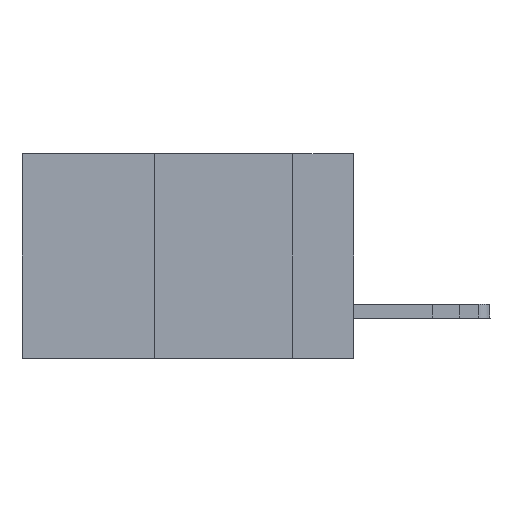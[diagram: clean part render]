
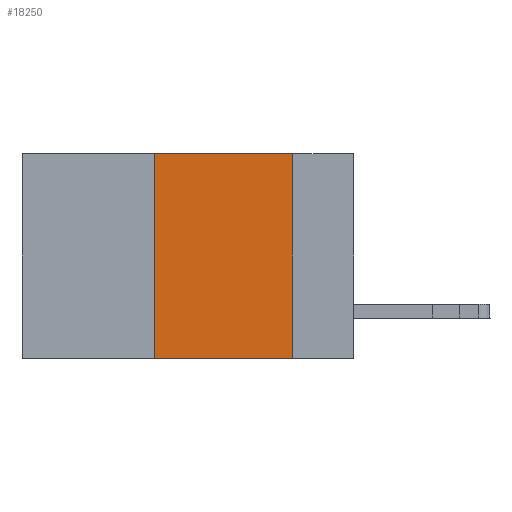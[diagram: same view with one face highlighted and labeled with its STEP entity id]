
A CAD part, left-side view. The second image highlights one B-rep face of the part: STEP entity #18250.
In plain terms, the highlighted planar face has unit normal (-1, 0, 0).
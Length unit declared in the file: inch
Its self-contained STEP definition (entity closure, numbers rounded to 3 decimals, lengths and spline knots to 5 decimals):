
#1842 = AXIS2_PLACEMENT_3D ( 'NONE', #34913, #21122, #20950 ) ;
#3930 = EDGE_CURVE ( 'NONE', #26078, #7096, #12836, .T. ) ;
#4949 = EDGE_CURVE ( 'NONE', #15551, #18416, #33529, .T. ) ;
#5114 = VECTOR ( 'NONE', #28613, 39.37008 ) ;
#7096 = VERTEX_POINT ( 'NONE', #31256 ) ;
#7903 = CARTESIAN_POINT ( 'NONE',  ( 0., 0.11, 0. ) ) ;
#8027 = VECTOR ( 'NONE', #15984, 39.37008 ) ;
#8038 = ORIENTED_EDGE ( 'NONE', *, *, #3930, .T. ) ;
#12127 = CARTESIAN_POINT ( 'NONE',  ( 0., 0.6, -0.37 ) ) ;
#12376 = DIRECTION ( 'NONE',  ( 0., 0., -1. ) ) ;
#12836 = LINE ( 'NONE', #12127, #24693 ) ;
#13246 = EDGE_LOOP ( 'NONE', ( #24107, #16454, #21526, #8038 ) ) ;
#15439 = CARTESIAN_POINT ( 'NONE',  ( 0., 0.11, 0. ) ) ;
#15551 = VERTEX_POINT ( 'NONE', #26642 ) ;
#15674 = PLANE ( 'NONE',  #1842 ) ;
#15984 = DIRECTION ( 'NONE',  ( 0., 0., 1. ) ) ;
#16454 = ORIENTED_EDGE ( 'NONE', *, *, #4949, .F. ) ;
#17394 = EDGE_CURVE ( 'NONE', #18416, #7096, #20714, .T. ) ;
#18250 = ADVANCED_FACE ( 'NONE', ( #31827 ), #15674, .F. ) ;
#18416 = VERTEX_POINT ( 'NONE', #7903 ) ;
#18526 = LINE ( 'NONE', #27226, #8027 ) ;
#20714 = LINE ( 'NONE', #15439, #32490 ) ;
#20950 = DIRECTION ( 'NONE',  ( 0., 0., -1. ) ) ;
#21122 = DIRECTION ( 'NONE',  ( 1., 0., 0. ) ) ;
#21526 = ORIENTED_EDGE ( 'NONE', *, *, #27087, .F. ) ;
#23174 = DIRECTION ( 'NONE',  ( 0., -1., 0. ) ) ;
#24107 = ORIENTED_EDGE ( 'NONE', *, *, #17394, .F. ) ;
#24693 = VECTOR ( 'NONE', #23174, 39.37008 ) ;
#25919 = CARTESIAN_POINT ( 'NONE',  ( 0., 0.36, -0.37 ) ) ;
#26078 = VERTEX_POINT ( 'NONE', #25919 ) ;
#26642 = CARTESIAN_POINT ( 'NONE',  ( 0., 0.36, 0. ) ) ;
#27087 = EDGE_CURVE ( 'NONE', #26078, #15551, #18526, .T. ) ;
#27226 = CARTESIAN_POINT ( 'NONE',  ( 0., 0.36, 0. ) ) ;
#28613 = DIRECTION ( 'NONE',  ( 0., -1., 0. ) ) ;
#30978 = CARTESIAN_POINT ( 'NONE',  ( 0., 0.6, 0. ) ) ;
#31256 = CARTESIAN_POINT ( 'NONE',  ( 0., 0.11, -0.37 ) ) ;
#31827 = FACE_OUTER_BOUND ( 'NONE', #13246, .T. ) ;
#32490 = VECTOR ( 'NONE', #12376, 39.37008 ) ;
#33529 = LINE ( 'NONE', #30978, #5114 ) ;
#34913 = CARTESIAN_POINT ( 'NONE',  ( 0., 0.6, 0. ) ) ;
